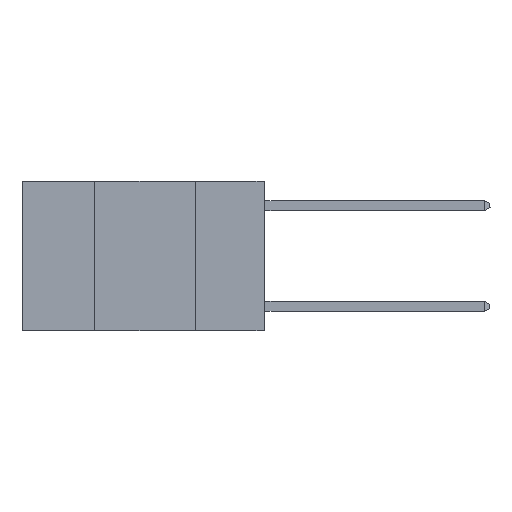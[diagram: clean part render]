
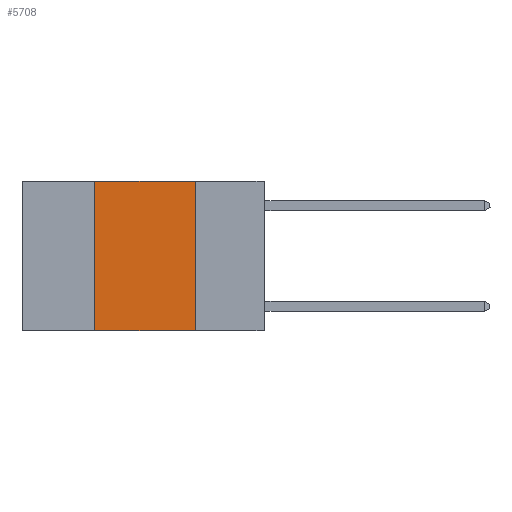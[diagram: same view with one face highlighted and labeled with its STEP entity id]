
A CAD part, left-side view. The second image highlights one B-rep face of the part: STEP entity #5708.
In plain terms, the highlighted planar face has unit normal (-1, 0, 0).
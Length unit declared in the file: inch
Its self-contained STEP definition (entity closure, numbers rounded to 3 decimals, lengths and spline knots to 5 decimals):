
#415 = PLANE ( 'NONE',  #11265 ) ;
#552 = CARTESIAN_POINT ( 'NONE',  ( 0., 0.42, -0.37 ) ) ;
#1160 = VERTEX_POINT ( 'NONE', #10939 ) ;
#1448 = LINE ( 'NONE', #1769, #11190 ) ;
#1651 = VERTEX_POINT ( 'NONE', #10701 ) ;
#1769 = CARTESIAN_POINT ( 'NONE',  ( 0., 0.6, 0. ) ) ;
#2757 = VECTOR ( 'NONE', #9215, 39.37008 ) ;
#3030 = LINE ( 'NONE', #8299, #7859 ) ;
#3306 = DIRECTION ( 'NONE',  ( 0., 0., -1. ) ) ;
#3711 = FACE_OUTER_BOUND ( 'NONE', #9291, .T. ) ;
#4337 = VERTEX_POINT ( 'NONE', #10688 ) ;
#4855 = VECTOR ( 'NONE', #5536, 39.37008 ) ;
#5052 = ORIENTED_EDGE ( 'NONE', *, *, #10092, .F. ) ;
#5424 = DIRECTION ( 'NONE',  ( 0., 0., 1. ) ) ;
#5470 = CARTESIAN_POINT ( 'NONE',  ( 0., 0.6, -0.37 ) ) ;
#5536 = DIRECTION ( 'NONE',  ( 0., 0., -1. ) ) ;
#5708 = ADVANCED_FACE ( 'NONE', ( #3711 ), #415, .F. ) ;
#5857 = ORIENTED_EDGE ( 'NONE', *, *, #9504, .F. ) ;
#6023 = ORIENTED_EDGE ( 'NONE', *, *, #7908, .F. ) ;
#6544 = VERTEX_POINT ( 'NONE', #552 ) ;
#7146 = CARTESIAN_POINT ( 'NONE',  ( 0., 0.6, 0. ) ) ;
#7171 = ORIENTED_EDGE ( 'NONE', *, *, #10105, .T. ) ;
#7859 = VECTOR ( 'NONE', #5424, 39.37008 ) ;
#7908 = EDGE_CURVE ( 'NONE', #1651, #1160, #1448, .T. ) ;
#8299 = CARTESIAN_POINT ( 'NONE',  ( 0., 0.42, 0. ) ) ;
#8998 = DIRECTION ( 'NONE',  ( 1., 0., 0. ) ) ;
#9215 = DIRECTION ( 'NONE',  ( 0., -1., 0. ) ) ;
#9291 = EDGE_LOOP ( 'NONE', ( #5857, #6023, #5052, #7171 ) ) ;
#9504 = EDGE_CURVE ( 'NONE', #1160, #4337, #11966, .T. ) ;
#10092 = EDGE_CURVE ( 'NONE', #6544, #1651, #3030, .T. ) ;
#10105 = EDGE_CURVE ( 'NONE', #6544, #4337, #10573, .T. ) ;
#10573 = LINE ( 'NONE', #5470, #2757 ) ;
#10688 = CARTESIAN_POINT ( 'NONE',  ( 0., 0.17, -0.37 ) ) ;
#10701 = CARTESIAN_POINT ( 'NONE',  ( 0., 0.42, 0. ) ) ;
#10939 = CARTESIAN_POINT ( 'NONE',  ( 0., 0.17, 0. ) ) ;
#11190 = VECTOR ( 'NONE', #12069, 39.37008 ) ;
#11265 = AXIS2_PLACEMENT_3D ( 'NONE', #7146, #8998, #3306 ) ;
#11966 = LINE ( 'NONE', #11977, #4855 ) ;
#11977 = CARTESIAN_POINT ( 'NONE',  ( 0., 0.17, 0. ) ) ;
#12069 = DIRECTION ( 'NONE',  ( 0., -1., 0. ) ) ;
